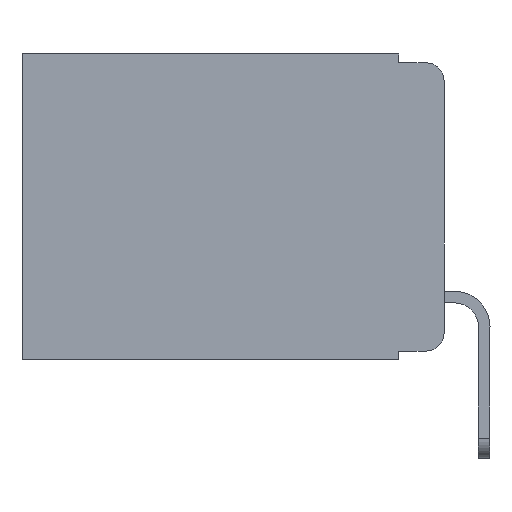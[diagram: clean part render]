
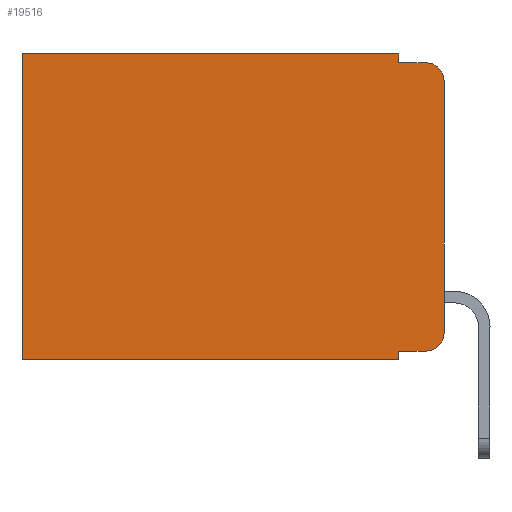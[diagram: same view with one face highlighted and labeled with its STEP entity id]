
A CAD part, left-side view. The second image highlights one B-rep face of the part: STEP entity #19516.
In plain terms, the highlighted planar face has unit normal (-1, 0, 0).
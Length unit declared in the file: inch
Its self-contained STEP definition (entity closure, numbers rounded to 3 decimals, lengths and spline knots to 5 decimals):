
#108 = AXIS2_PLACEMENT_3D ( 'NONE', #18960, #10056, #9969 ) ;
#362 = DIRECTION ( 'NONE',  ( 0., 1., 0. ) ) ;
#749 = LINE ( 'NONE', #14098, #18776 ) ;
#861 = VECTOR ( 'NONE', #17944, 39.37008 ) ;
#882 = VERTEX_POINT ( 'NONE', #13620 ) ;
#1045 = LINE ( 'NONE', #4649, #12882 ) ;
#1932 = LINE ( 'NONE', #18257, #12638 ) ;
#2082 = CARTESIAN_POINT ( 'NONE',  ( 0.298, 0., 0. ) ) ;
#2184 = ORIENTED_EDGE ( 'NONE', *, *, #22507, .T. ) ;
#2391 = EDGE_CURVE ( 'NONE', #882, #6466, #8822, .T. ) ;
#2856 = CARTESIAN_POINT ( 'NONE',  ( 0.298, 0., -0.03 ) ) ;
#3123 = EDGE_LOOP ( 'NONE', ( #8291, #10878, #14960, #18335, #14495, #2184, #15083, #17377, #16450, #20275 ) ) ;
#3262 = CARTESIAN_POINT ( 'NONE',  ( 0.298, 0.051, -0.01 ) ) ;
#3629 = VERTEX_POINT ( 'NONE', #18034 ) ;
#4649 = CARTESIAN_POINT ( 'NONE',  ( 0.298, 0., 0. ) ) ;
#6319 = CARTESIAN_POINT ( 'NONE',  ( 0.298, 0.051, 0. ) ) ;
#6466 = VERTEX_POINT ( 'NONE', #23084 ) ;
#6683 = VERTEX_POINT ( 'NONE', #12681 ) ;
#8130 = CARTESIAN_POINT ( 'NONE',  ( 0.298, 0.051, 0. ) ) ;
#8291 = ORIENTED_EDGE ( 'NONE', *, *, #10504, .F. ) ;
#8618 = FACE_OUTER_BOUND ( 'NONE', #3123, .T. ) ;
#8772 = CIRCLE ( 'NONE', #12438, 0.02 ) ;
#8816 = DIRECTION ( 'NONE',  ( 0., -1., 0. ) ) ;
#8822 = LINE ( 'NONE', #3262, #15899 ) ;
#8962 = CARTESIAN_POINT ( 'NONE',  ( 0.298, 0.473, 0. ) ) ;
#9655 = LINE ( 'NONE', #17952, #22084 ) ;
#9900 = EDGE_CURVE ( 'NONE', #12620, #21185, #1932, .T. ) ;
#9955 = DIRECTION ( 'NONE',  ( 0., 0., -1. ) ) ;
#9969 = DIRECTION ( 'NONE',  ( 0., 0., -1. ) ) ;
#10056 = DIRECTION ( 'NONE',  ( 1., 0., 0. ) ) ;
#10199 = DIRECTION ( 'NONE',  ( -1., 0., 0. ) ) ;
#10498 = DIRECTION ( 'NONE',  ( 0., -1., 0. ) ) ;
#10504 = EDGE_CURVE ( 'NONE', #14405, #3629, #13149, .T. ) ;
#10779 = VERTEX_POINT ( 'NONE', #8130 ) ;
#10844 = VECTOR ( 'NONE', #9955, 39.37008 ) ;
#10878 = ORIENTED_EDGE ( 'NONE', *, *, #15846, .T. ) ;
#11055 = EDGE_CURVE ( 'NONE', #11975, #15268, #749, .T. ) ;
#11975 = VERTEX_POINT ( 'NONE', #15347 ) ;
#12014 = DIRECTION ( 'NONE',  ( 0., 0., -1. ) ) ;
#12060 = DIRECTION ( 'NONE',  ( 0., 1., 0. ) ) ;
#12356 = CARTESIAN_POINT ( 'NONE',  ( 0.298, 0.473, -0.343 ) ) ;
#12438 = AXIS2_PLACEMENT_3D ( 'NONE', #17293, #10199, #12014 ) ;
#12532 = EDGE_CURVE ( 'NONE', #15268, #3629, #22439, .T. ) ;
#12620 = VERTEX_POINT ( 'NONE', #17139 ) ;
#12638 = VECTOR ( 'NONE', #362, 39.37008 ) ;
#12681 = CARTESIAN_POINT ( 'NONE',  ( 0.298, 0.473, 0. ) ) ;
#12882 = VECTOR ( 'NONE', #12060, 39.37008 ) ;
#13149 = LINE ( 'NONE', #2082, #14266 ) ;
#13336 = CARTESIAN_POINT ( 'NONE',  ( 0.298, 0.02, -0.313 ) ) ;
#13569 = AXIS2_PLACEMENT_3D ( 'NONE', #13336, #16666, #20361 ) ;
#13620 = CARTESIAN_POINT ( 'NONE',  ( 0.298, 0.051, -0.01 ) ) ;
#14098 = CARTESIAN_POINT ( 'NONE',  ( 0.298, 0.051, -0.333 ) ) ;
#14266 = VECTOR ( 'NONE', #14424, 39.37008 ) ;
#14356 = LINE ( 'NONE', #8962, #861 ) ;
#14405 = VERTEX_POINT ( 'NONE', #2856 ) ;
#14424 = DIRECTION ( 'NONE',  ( 0., 0., -1. ) ) ;
#14495 = ORIENTED_EDGE ( 'NONE', *, *, #18955, .T. ) ;
#14681 = EDGE_CURVE ( 'NONE', #11975, #12620, #9655, .T. ) ;
#14960 = ORIENTED_EDGE ( 'NONE', *, *, #2391, .F. ) ;
#15083 = ORIENTED_EDGE ( 'NONE', *, *, #9900, .F. ) ;
#15268 = VERTEX_POINT ( 'NONE', #23057 ) ;
#15347 = CARTESIAN_POINT ( 'NONE',  ( 0.298, 0.051, -0.333 ) ) ;
#15846 = EDGE_CURVE ( 'NONE', #14405, #6466, #8772, .T. ) ;
#15899 = VECTOR ( 'NONE', #10498, 39.37008 ) ;
#15924 = DIRECTION ( 'NONE',  ( 0., 0., -1. ) ) ;
#16450 = ORIENTED_EDGE ( 'NONE', *, *, #11055, .T. ) ;
#16666 = DIRECTION ( 'NONE',  ( -1., 0., 0. ) ) ;
#17139 = CARTESIAN_POINT ( 'NONE',  ( 0.298, 0.051, -0.343 ) ) ;
#17293 = CARTESIAN_POINT ( 'NONE',  ( 0.298, 0.02, -0.03 ) ) ;
#17377 = ORIENTED_EDGE ( 'NONE', *, *, #14681, .F. ) ;
#17944 = DIRECTION ( 'NONE',  ( 0., 0., -1. ) ) ;
#17952 = CARTESIAN_POINT ( 'NONE',  ( 0.298, 0.051, 0. ) ) ;
#18034 = CARTESIAN_POINT ( 'NONE',  ( 0.298, 0., -0.313 ) ) ;
#18257 = CARTESIAN_POINT ( 'NONE',  ( 0.298, 0., -0.343 ) ) ;
#18335 = ORIENTED_EDGE ( 'NONE', *, *, #20015, .F. ) ;
#18776 = VECTOR ( 'NONE', #8816, 39.37008 ) ;
#18955 = EDGE_CURVE ( 'NONE', #10779, #6683, #1045, .T. ) ;
#18960 = CARTESIAN_POINT ( 'NONE',  ( 0.298, 0., 0. ) ) ;
#19516 = ADVANCED_FACE ( 'NONE', ( #8618 ), #20693, .F. ) ;
#20015 = EDGE_CURVE ( 'NONE', #10779, #882, #20162, .T. ) ;
#20162 = LINE ( 'NONE', #6319, #10844 ) ;
#20275 = ORIENTED_EDGE ( 'NONE', *, *, #12532, .T. ) ;
#20361 = DIRECTION ( 'NONE',  ( 0., 0., -1. ) ) ;
#20693 = PLANE ( 'NONE',  #108 ) ;
#21185 = VERTEX_POINT ( 'NONE', #12356 ) ;
#22084 = VECTOR ( 'NONE', #15924, 39.37008 ) ;
#22439 = CIRCLE ( 'NONE', #13569, 0.02 ) ;
#22507 = EDGE_CURVE ( 'NONE', #6683, #21185, #14356, .T. ) ;
#23057 = CARTESIAN_POINT ( 'NONE',  ( 0.298, 0.02, -0.333 ) ) ;
#23084 = CARTESIAN_POINT ( 'NONE',  ( 0.298, 0.02, -0.01 ) ) ;
